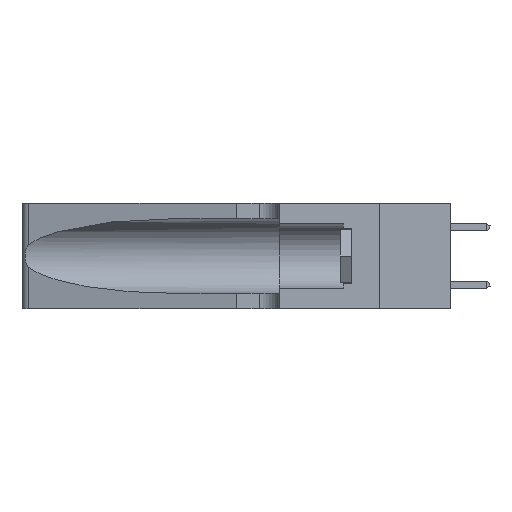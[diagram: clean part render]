
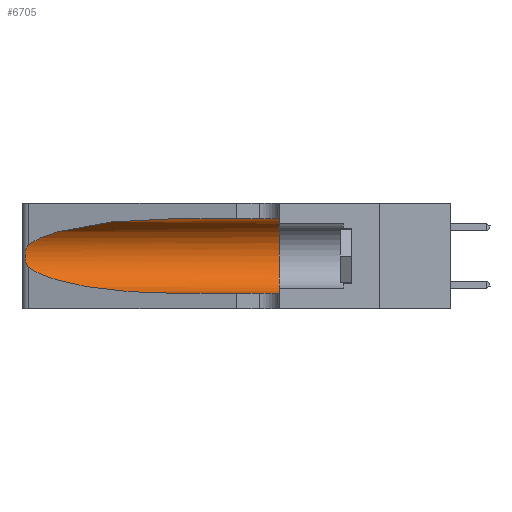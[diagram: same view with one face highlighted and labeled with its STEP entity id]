
A CAD part, left-side view. The second image highlights one B-rep face of the part: STEP entity #6705.
In plain terms, the highlighted cylindrical face has radius 3.308 mm (diameter 6.617 mm), a partial arc.
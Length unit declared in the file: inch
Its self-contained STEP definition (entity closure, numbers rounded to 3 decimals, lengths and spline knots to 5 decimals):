
#646 = DIRECTION ( 'NONE',  ( 0., 1., 0. ) ) ;
#718 = CARTESIAN_POINT ( 'NONE',  ( 0.25787, 1.23484, 0.2124 ) ) ;
#1438 = ORIENTED_EDGE ( 'NONE', *, *, #34179, .T. ) ;
#2457 = VERTEX_POINT ( 'NONE', #20878 ) ;
#2520 = CARTESIAN_POINT ( 'NONE',  ( 0.25487, 1.22718, 0.14631 ) ) ;
#2629 = CARTESIAN_POINT ( 'NONE',  ( 0.1305, 0.72297, 0.05475 ) ) ;
#2694 = DIRECTION ( 'NONE',  ( 0., -1., 0. ) ) ;
#3506 = CARTESIAN_POINT ( 'NONE',  ( 0.26018, 1.23835, 0.19895 ) ) ;
#3635 = AXIS2_PLACEMENT_3D ( 'NONE', #12368, #17628, #25561 ) ;
#4196 = VECTOR ( 'NONE', #2694, 39.37008 ) ;
#4240 = FACE_OUTER_BOUND ( 'NONE', #20299, .T. ) ;
#4568 = EDGE_CURVE ( 'NONE', #7006, #14937, #22364, .T. ) ;
#5288 = EDGE_CURVE ( 'NONE', #15465, #7967, #31758, .T. ) ;
#5944 = ORIENTED_EDGE ( 'NONE', *, *, #5288, .T. ) ;
#6086 = CARTESIAN_POINT ( 'NONE',  ( 0.25555, 1.22994, 0.2215 ) ) ;
#6207 = CARTESIAN_POINT ( 'NONE',  ( 0.26075, 1.23896, 0.178 ) ) ;
#6705 = ADVANCED_FACE ( 'NONE', ( #4240 ), #17663, .F. ) ;
#7006 = VERTEX_POINT ( 'NONE', #31930 ) ;
#7866 = EDGE_CURVE ( 'NONE', #11580, #7006, #18006, .T. ) ;
#7967 = VERTEX_POINT ( 'NONE', #23223 ) ;
#8916 = CARTESIAN_POINT ( 'NONE',  ( 0.25856, 1.23593, 0.16098 ) ) ;
#10061 = CARTESIAN_POINT ( 'NONE',  ( 0.25487, 1.22718, 0.22369 ) ) ;
#10654 = CARTESIAN_POINT ( 'NONE',  ( 0.2373, 1.15595, 0.08982 ) ) ;
#10817 =( BOUNDED_CURVE ( )  B_SPLINE_CURVE ( 3, ( #2520, #10654, #18730, #2629 ),
 .UNSPECIFIED., .F., .F. ) 
 B_SPLINE_CURVE_WITH_KNOTS ( ( 4, 4 ),
 ( 3.44316, 4.71239 ),
 .UNSPECIFIED. ) 
 CURVE ( )  GEOMETRIC_REPRESENTATION_ITEM ( )  RATIONAL_B_SPLINE_CURVE ( ( 1., 0.87, 0.87, 1. ) ) 
 REPRESENTATION_ITEM ( '' )  );
#11106 = CARTESIAN_POINT ( 'NONE',  ( 0.1305, 0.72297, 0.31525 ) ) ;
#11306 = EDGE_CURVE ( 'NONE', #11580, #15465, #13397, .T. ) ;
#11580 = VERTEX_POINT ( 'NONE', #11106 ) ;
#11629 = CARTESIAN_POINT ( 'NONE',  ( 0.25639, 1.23186, 0.15144 ) ) ;
#12368 = CARTESIAN_POINT ( 'NONE',  ( 0.1305, 1.61858, 0.185 ) ) ;
#12552 = ORIENTED_EDGE ( 'NONE', *, *, #7866, .F. ) ;
#13397 =( BOUNDED_CURVE ( )  B_SPLINE_CURVE ( 3, ( #23294, #20682, #25946, #10061 ),
 .UNSPECIFIED., .F., .F. ) 
 B_SPLINE_CURVE_WITH_KNOTS ( ( 4, 4 ),
 ( 1.5708, 2.84003 ),
 .UNSPECIFIED. ) 
 CURVE ( )  GEOMETRIC_REPRESENTATION_ITEM ( )  RATIONAL_B_SPLINE_CURVE ( ( 1., 0.87, 0.87, 1. ) ) 
 REPRESENTATION_ITEM ( '' )  );
#13909 = CARTESIAN_POINT ( 'NONE',  ( 0.25487, 1.22718, 0.22369 ) ) ;
#14186 = CARTESIAN_POINT ( 'NONE',  ( 0.25639, 1.23184, 0.21858 ) ) ;
#14298 = CARTESIAN_POINT ( 'NONE',  ( 0.25487, 1.22718, 0.14631 ) ) ;
#14937 = VERTEX_POINT ( 'NONE', #22308 ) ;
#15465 = VERTEX_POINT ( 'NONE', #13909 ) ;
#16082 = CARTESIAN_POINT ( 'NONE',  ( 0.1305, 1.61858, 0.05475 ) ) ;
#16817 = CARTESIAN_POINT ( 'NONE',  ( 0.1305, 0.35, 0.185 ) ) ;
#16898 = CARTESIAN_POINT ( 'NONE',  ( 0.25487, 1.22718, 0.22369 ) ) ;
#17628 = DIRECTION ( 'NONE',  ( 0., -1., 0. ) ) ;
#17663 = CYLINDRICAL_SURFACE ( 'NONE', #3635, 0.13025 ) ;
#18006 = LINE ( 'NONE', #20151, #31939 ) ;
#18730 = CARTESIAN_POINT ( 'NONE',  ( 0.18966, 0.96281, 0.05475 ) ) ;
#19476 = DIRECTION ( 'NONE',  ( 0., 0., 1. ) ) ;
#19554 = CARTESIAN_POINT ( 'NONE',  ( 0.25854, 1.2359, 0.20912 ) ) ;
#20151 = CARTESIAN_POINT ( 'NONE',  ( 0.1305, 1.61858, 0.31525 ) ) ;
#20299 = EDGE_LOOP ( 'NONE', ( #25774, #5944, #1438, #20672, #25735, #12552 ) ) ;
#20672 = ORIENTED_EDGE ( 'NONE', *, *, #22114, .T. ) ;
#20682 = CARTESIAN_POINT ( 'NONE',  ( 0.18966, 0.96281, 0.31525 ) ) ;
#20871 = AXIS2_PLACEMENT_3D ( 'NONE', #16817, #646, #19476 ) ;
#20878 = CARTESIAN_POINT ( 'NONE',  ( 0.1305, 0.72297, 0.05475 ) ) ;
#22114 = EDGE_CURVE ( 'NONE', #2457, #14937, #32403, .T. ) ;
#22196 = CARTESIAN_POINT ( 'NONE',  ( 0.26075, 1.23896, 0.19203 ) ) ;
#22308 = CARTESIAN_POINT ( 'NONE',  ( 0.1305, 0.35, 0.05475 ) ) ;
#22364 = CIRCLE ( 'NONE', #20871, 0.13025 ) ;
#22778 = DIRECTION ( 'NONE',  ( 0., -1., 0. ) ) ;
#23223 = CARTESIAN_POINT ( 'NONE',  ( 0.25487, 1.22718, 0.14631 ) ) ;
#23294 = CARTESIAN_POINT ( 'NONE',  ( 0.1305, 0.72297, 0.31525 ) ) ;
#24841 = CARTESIAN_POINT ( 'NONE',  ( 0.26017, 1.23833, 0.17102 ) ) ;
#25561 = DIRECTION ( 'NONE',  ( 0., 0., -1. ) ) ;
#25735 = ORIENTED_EDGE ( 'NONE', *, *, #4568, .F. ) ;
#25774 = ORIENTED_EDGE ( 'NONE', *, *, #11306, .T. ) ;
#25946 = CARTESIAN_POINT ( 'NONE',  ( 0.2373, 1.15595, 0.28018 ) ) ;
#27477 = CARTESIAN_POINT ( 'NONE',  ( 0.25789, 1.23486, 0.15765 ) ) ;
#30101 = CARTESIAN_POINT ( 'NONE',  ( 0.25555, 1.22993, 0.14849 ) ) ;
#31758 = B_SPLINE_CURVE_WITH_KNOTS ( 'NONE', 3,
 ( #16898, #6086, #14186, #718, #19554, #3506, #22196, #6207, #24841, #8916, #27477, #11629, #30101, #14298 ),
 .UNSPECIFIED., .F., .F.,
 ( 4, 2, 2, 2, 2, 2, 4 ),
 ( 0., 0.00027, 0.00053, 0.00107, 0.0016, 0.00187, 0.00214 ),
 .UNSPECIFIED. ) ;
#31930 = CARTESIAN_POINT ( 'NONE',  ( 0.1305, 0.35, 0.31525 ) ) ;
#31939 = VECTOR ( 'NONE', #22778, 39.37008 ) ;
#32403 = LINE ( 'NONE', #16082, #4196 ) ;
#34179 = EDGE_CURVE ( 'NONE', #7967, #2457, #10817, .T. ) ;
